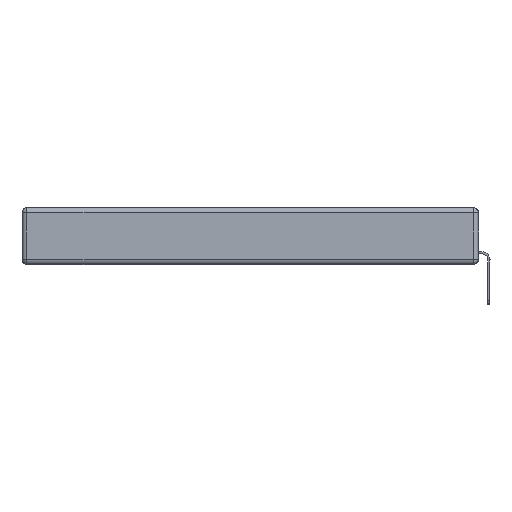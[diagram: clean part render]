
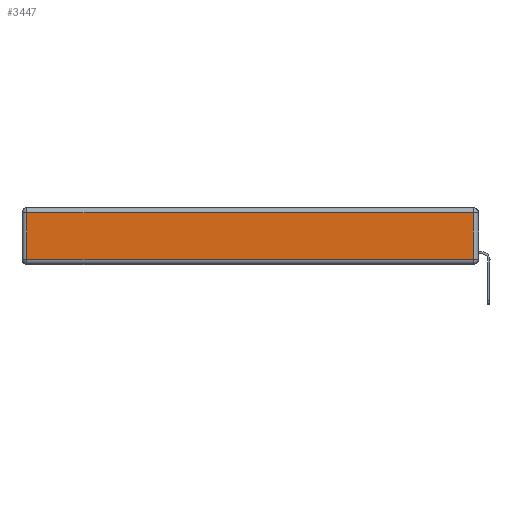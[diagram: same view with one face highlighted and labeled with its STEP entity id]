
A CAD part, left-side view. The second image highlights one B-rep face of the part: STEP entity #3447.
In plain terms, the highlighted planar face has unit normal (-1, 0, 0).
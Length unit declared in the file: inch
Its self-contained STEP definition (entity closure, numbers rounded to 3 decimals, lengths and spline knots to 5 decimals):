
#13 = DIRECTION ( 'NONE',  ( 0., -1., 0. ) ) ;
#1910 = CARTESIAN_POINT ( 'NONE',  ( 0., 0.03, -0.313 ) ) ;
#2654 = VECTOR ( 'NONE', #3357, 39.37008 ) ;
#3357 = DIRECTION ( 'NONE',  ( 0., 1., 0. ) ) ;
#3447 = ADVANCED_FACE ( 'NONE', ( #14841 ), #16583, .T. ) ;
#4285 = LINE ( 'NONE', #8283, #13873 ) ;
#4713 = ORIENTED_EDGE ( 'NONE', *, *, #11781, .T. ) ;
#4770 = CARTESIAN_POINT ( 'NONE',  ( 0., 2.72, -0.343 ) ) ;
#5097 = LINE ( 'NONE', #5231, #2654 ) ;
#5231 = CARTESIAN_POINT ( 'NONE',  ( 0., 2.75, -0.03 ) ) ;
#6592 = CARTESIAN_POINT ( 'NONE',  ( 0., 2.72, -0.313 ) ) ;
#7130 = EDGE_CURVE ( 'NONE', #8612, #19425, #4285, .T. ) ;
#7545 = VERTEX_POINT ( 'NONE', #18416 ) ;
#8283 = CARTESIAN_POINT ( 'NONE',  ( 0., 0., -0.313 ) ) ;
#8286 = DIRECTION ( 'NONE',  ( 0., 0., 1. ) ) ;
#8612 = VERTEX_POINT ( 'NONE', #6592 ) ;
#11781 = EDGE_CURVE ( 'NONE', #19425, #7545, #21679, .T. ) ;
#13658 = ORIENTED_EDGE ( 'NONE', *, *, #14226, .T. ) ;
#13873 = VECTOR ( 'NONE', #13, 39.37008 ) ;
#14226 = EDGE_CURVE ( 'NONE', #17891, #8612, #14389, .T. ) ;
#14369 = ORIENTED_EDGE ( 'NONE', *, *, #26121, .T. ) ;
#14389 = LINE ( 'NONE', #4770, #22964 ) ;
#14841 = FACE_OUTER_BOUND ( 'NONE', #16810, .T. ) ;
#16583 = PLANE ( 'NONE',  #25258 ) ;
#16810 = EDGE_LOOP ( 'NONE', ( #22819, #4713, #14369, #13658 ) ) ;
#17891 = VERTEX_POINT ( 'NONE', #18629 ) ;
#18416 = CARTESIAN_POINT ( 'NONE',  ( 0., 0.03, -0.03 ) ) ;
#18629 = CARTESIAN_POINT ( 'NONE',  ( 0., 2.72, -0.03 ) ) ;
#19425 = VERTEX_POINT ( 'NONE', #1910 ) ;
#20843 = CARTESIAN_POINT ( 'NONE',  ( 0., 0., -0.343 ) ) ;
#21679 = LINE ( 'NONE', #23561, #24990 ) ;
#22586 = DIRECTION ( 'NONE',  ( -1., 0., 0. ) ) ;
#22819 = ORIENTED_EDGE ( 'NONE', *, *, #7130, .T. ) ;
#22964 = VECTOR ( 'NONE', #24675, 39.37008 ) ;
#23561 = CARTESIAN_POINT ( 'NONE',  ( 0., 0.03, -0.343 ) ) ;
#24675 = DIRECTION ( 'NONE',  ( 0., 0., -1. ) ) ;
#24990 = VECTOR ( 'NONE', #25574, 39.37008 ) ;
#25258 = AXIS2_PLACEMENT_3D ( 'NONE', #20843, #22586, #8286 ) ;
#25574 = DIRECTION ( 'NONE',  ( 0., 0., 1. ) ) ;
#26121 = EDGE_CURVE ( 'NONE', #7545, #17891, #5097, .T. ) ;
